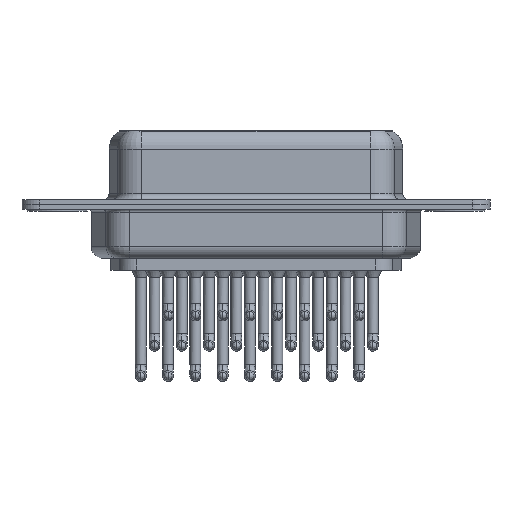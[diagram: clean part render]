
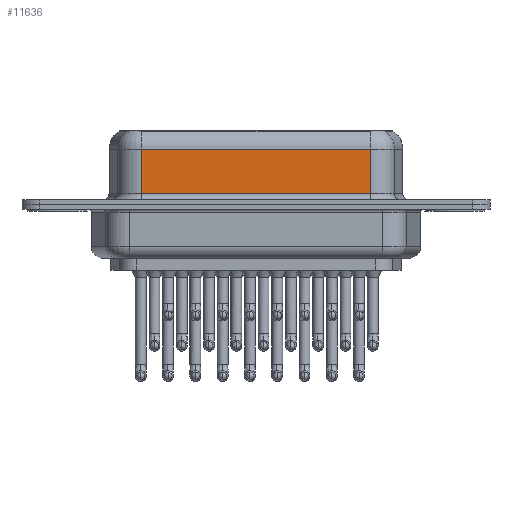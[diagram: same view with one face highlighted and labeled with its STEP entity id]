
A CAD part, front view. The second image highlights one B-rep face of the part: STEP entity #11636.
In plain terms, the highlighted planar face has unit normal (0, -1, 0).
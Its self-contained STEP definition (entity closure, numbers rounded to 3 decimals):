
#330 = FACE_OUTER_BOUND ( 'NONE', #17525, .T. ) ;
#3245 = EDGE_CURVE ( 'NONE', #16611, #15813, #6323, .T. ) ;
#3982 = LINE ( 'NONE', #7639, #21401 ) ;
#5606 = DIRECTION ( 'NONE',  ( -1., 0., 0. ) ) ;
#6303 = VECTOR ( 'NONE', #5606, 1000. ) ;
#6323 = LINE ( 'NONE', #16926, #10295 ) ;
#6435 = VECTOR ( 'NONE', #7263, 1000. ) ;
#7263 = DIRECTION ( 'NONE',  ( 1., 0., 0. ) ) ;
#7639 = CARTESIAN_POINT ( 'NONE',  ( 26.262, -3.95, 6.4 ) ) ;
#8500 = ORIENTED_EDGE ( 'NONE', *, *, #15198, .F. ) ;
#8817 = CARTESIAN_POINT ( 'NONE',  ( 26.262, -3.95, 0.9 ) ) ;
#8965 = CARTESIAN_POINT ( 'NONE',  ( 26.262, -3.95, 0.9 ) ) ;
#10295 = VECTOR ( 'NONE', #17148, 1000. ) ;
#10746 = CARTESIAN_POINT ( 'NONE',  ( 26.262, -3.95, 4.65 ) ) ;
#11527 = EDGE_CURVE ( 'NONE', #15813, #20069, #15966, .T. ) ;
#11636 = ADVANCED_FACE ( 'NONE', ( #330 ), #21778, .F. ) ;
#11723 = DIRECTION ( 'NONE',  ( -1., 0., 0. ) ) ;
#13353 = CARTESIAN_POINT ( 'NONE',  ( 26.262, -3.95, 6.4 ) ) ;
#14324 = AXIS2_PLACEMENT_3D ( 'NONE', #13353, #21842, #11723 ) ;
#14443 = CARTESIAN_POINT ( 'NONE',  ( 7.038, -3.95, 4.65 ) ) ;
#15198 = EDGE_CURVE ( 'NONE', #17377, #20069, #3982, .T. ) ;
#15813 = VERTEX_POINT ( 'NONE', #19067 ) ;
#15826 = LINE ( 'NONE', #10746, #6303 ) ;
#15877 = EDGE_CURVE ( 'NONE', #17377, #16611, #15826, .T. ) ;
#15966 = LINE ( 'NONE', #8965, #6435 ) ;
#16129 = DIRECTION ( 'NONE',  ( 0., 0., -1. ) ) ;
#16611 = VERTEX_POINT ( 'NONE', #14443 ) ;
#16888 = CARTESIAN_POINT ( 'NONE',  ( 26.262, -3.95, 4.65 ) ) ;
#16926 = CARTESIAN_POINT ( 'NONE',  ( 7.038, -3.95, 6.4 ) ) ;
#17148 = DIRECTION ( 'NONE',  ( 0., 0., -1. ) ) ;
#17377 = VERTEX_POINT ( 'NONE', #16888 ) ;
#17438 = ORIENTED_EDGE ( 'NONE', *, *, #15877, .T. ) ;
#17525 = EDGE_LOOP ( 'NONE', ( #8500, #17438, #21381, #19194 ) ) ;
#19067 = CARTESIAN_POINT ( 'NONE',  ( 7.038, -3.95, 0.9 ) ) ;
#19194 = ORIENTED_EDGE ( 'NONE', *, *, #11527, .T. ) ;
#20069 = VERTEX_POINT ( 'NONE', #8817 ) ;
#21381 = ORIENTED_EDGE ( 'NONE', *, *, #3245, .T. ) ;
#21401 = VECTOR ( 'NONE', #16129, 1000. ) ;
#21778 = PLANE ( 'NONE',  #14324 ) ;
#21842 = DIRECTION ( 'NONE',  ( 0., 1., 0. ) ) ;
